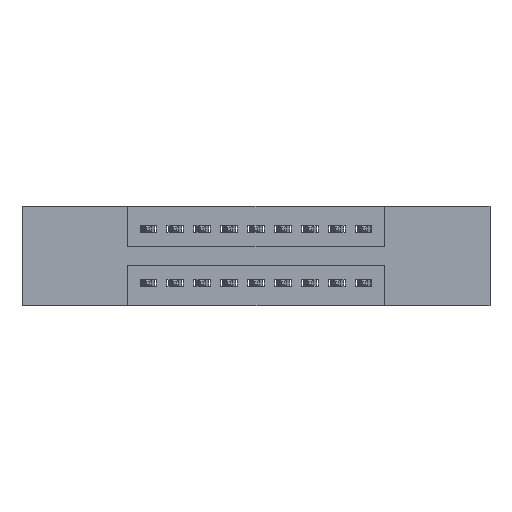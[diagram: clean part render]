
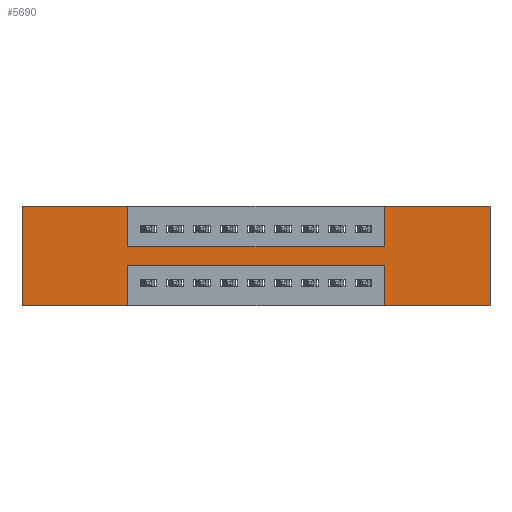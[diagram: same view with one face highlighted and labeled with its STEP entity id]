
A CAD part, front view. The second image highlights one B-rep face of the part: STEP entity #5690.
In plain terms, the highlighted planar face has unit normal (0, -1, 0).
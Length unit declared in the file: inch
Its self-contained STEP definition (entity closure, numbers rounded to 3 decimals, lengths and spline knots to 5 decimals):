
#27 = EDGE_CURVE ( 'NONE', #7362, #11286, #8275, .T. ) ;
#112 = VERTEX_POINT ( 'NONE', #4151 ) ;
#224 = LINE ( 'NONE', #10759, #5105 ) ;
#239 = VECTOR ( 'NONE', #3613, 39.37008 ) ;
#330 = LINE ( 'NONE', #7866, #8213 ) ;
#507 = CARTESIAN_POINT ( 'NONE',  ( 1.735, 0., -0.37 ) ) ;
#945 = VERTEX_POINT ( 'NONE', #2384 ) ;
#1227 = VERTEX_POINT ( 'NONE', #5487 ) ;
#1236 = ORIENTED_EDGE ( 'NONE', *, *, #6368, .F. ) ;
#1239 = LINE ( 'NONE', #10356, #7208 ) ;
#1295 = ORIENTED_EDGE ( 'NONE', *, *, #3933, .F. ) ;
#1447 = DIRECTION ( 'NONE',  ( -1., 0., 0. ) ) ;
#1628 = ORIENTED_EDGE ( 'NONE', *, *, #2714, .F. ) ;
#1631 = ORIENTED_EDGE ( 'NONE', *, *, #1986, .F. ) ;
#1646 = DIRECTION ( 'NONE',  ( 0., -1., 0. ) ) ;
#1829 = ORIENTED_EDGE ( 'NONE', *, *, #4329, .F. ) ;
#1986 = EDGE_CURVE ( 'NONE', #8914, #5612, #5753, .T. ) ;
#2113 = EDGE_CURVE ( 'NONE', #112, #8914, #330, .T. ) ;
#2194 = ORIENTED_EDGE ( 'NONE', *, *, #6553, .F. ) ;
#2314 = CARTESIAN_POINT ( 'NONE',  ( 0., 0., 0. ) ) ;
#2384 = CARTESIAN_POINT ( 'NONE',  ( 0.3925, 0., 0. ) ) ;
#2404 = CARTESIAN_POINT ( 'NONE',  ( 0., 0., 0. ) ) ;
#2482 = LINE ( 'NONE', #10685, #239 ) ;
#2489 = FACE_OUTER_BOUND ( 'NONE', #9531, .T. ) ;
#2555 = CARTESIAN_POINT ( 'NONE',  ( 1.3425, 0., -0.37 ) ) ;
#2714 = EDGE_CURVE ( 'NONE', #10929, #112, #3242, .T. ) ;
#2785 = VECTOR ( 'NONE', #1447, 39.37008 ) ;
#2789 = VERTEX_POINT ( 'NONE', #3865 ) ;
#2868 = ORIENTED_EDGE ( 'NONE', *, *, #27, .F. ) ;
#3043 = VECTOR ( 'NONE', #5498, 39.37008 ) ;
#3101 = CARTESIAN_POINT ( 'NONE',  ( 0.3925, 0., -0.22 ) ) ;
#3113 = CARTESIAN_POINT ( 'NONE',  ( 0., 0., -0.37 ) ) ;
#3242 = LINE ( 'NONE', #5253, #9728 ) ;
#3300 = DIRECTION ( 'NONE',  ( 0., 0., -1. ) ) ;
#3613 = DIRECTION ( 'NONE',  ( 0., 0., 1. ) ) ;
#3855 = ORIENTED_EDGE ( 'NONE', *, *, #9742, .F. ) ;
#3865 = CARTESIAN_POINT ( 'NONE',  ( 0.3925, 0., -0.15 ) ) ;
#3933 = EDGE_CURVE ( 'NONE', #945, #2789, #1239, .T. ) ;
#4038 = CARTESIAN_POINT ( 'NONE',  ( 0., 0., 0. ) ) ;
#4043 = LINE ( 'NONE', #9904, #5548 ) ;
#4151 = CARTESIAN_POINT ( 'NONE',  ( 0.3925, 0., -0.37 ) ) ;
#4329 = EDGE_CURVE ( 'NONE', #4394, #5399, #9144, .T. ) ;
#4394 = VERTEX_POINT ( 'NONE', #2555 ) ;
#4529 = EDGE_CURVE ( 'NONE', #5612, #945, #5687, .T. ) ;
#4893 = EDGE_CURVE ( 'NONE', #5399, #10929, #5140, .T. ) ;
#5105 = VECTOR ( 'NONE', #9064, 39.37008 ) ;
#5140 = LINE ( 'NONE', #10385, #2785 ) ;
#5190 = DIRECTION ( 'NONE',  ( 0., 0., 1. ) ) ;
#5253 = CARTESIAN_POINT ( 'NONE',  ( 0.3925, 0., -0.37 ) ) ;
#5386 = CARTESIAN_POINT ( 'NONE',  ( 1.735, 0., 0. ) ) ;
#5399 = VERTEX_POINT ( 'NONE', #8584 ) ;
#5487 = CARTESIAN_POINT ( 'NONE',  ( 1.3425, 0., -0.15 ) ) ;
#5498 = DIRECTION ( 'NONE',  ( 1., 0., 0. ) ) ;
#5548 = VECTOR ( 'NONE', #8063, 39.37008 ) ;
#5612 = VERTEX_POINT ( 'NONE', #4038 ) ;
#5619 = DIRECTION ( 'NONE',  ( 0., 0., 1. ) ) ;
#5687 = LINE ( 'NONE', #2314, #8302 ) ;
#5690 = ADVANCED_FACE ( 'NONE', ( #2489 ), #11340, .T. ) ;
#5753 = LINE ( 'NONE', #2404, #6993 ) ;
#6368 = EDGE_CURVE ( 'NONE', #1227, #7362, #2482, .T. ) ;
#6553 = EDGE_CURVE ( 'NONE', #9097, #4394, #224, .T. ) ;
#6993 = VECTOR ( 'NONE', #5190, 39.37008 ) ;
#7103 = DIRECTION ( 'NONE',  ( 1., 0., 0. ) ) ;
#7208 = VECTOR ( 'NONE', #3300, 39.37008 ) ;
#7300 = CARTESIAN_POINT ( 'NONE',  ( 1.3425, 0., -0.37 ) ) ;
#7362 = VERTEX_POINT ( 'NONE', #10953 ) ;
#7866 = CARTESIAN_POINT ( 'NONE',  ( 0., 0., -0.37 ) ) ;
#8063 = DIRECTION ( 'NONE',  ( 0., 0., -1. ) ) ;
#8213 = VECTOR ( 'NONE', #9744, 39.37008 ) ;
#8275 = LINE ( 'NONE', #8725, #3043 ) ;
#8302 = VECTOR ( 'NONE', #8568, 39.37008 ) ;
#8515 = ORIENTED_EDGE ( 'NONE', *, *, #4893, .F. ) ;
#8568 = DIRECTION ( 'NONE',  ( 1., 0., 0. ) ) ;
#8584 = CARTESIAN_POINT ( 'NONE',  ( 1.3425, 0., -0.22 ) ) ;
#8654 = EDGE_CURVE ( 'NONE', #11286, #9097, #4043, .T. ) ;
#8697 = CARTESIAN_POINT ( 'NONE',  ( 0., 0., -0.37 ) ) ;
#8725 = CARTESIAN_POINT ( 'NONE',  ( 0., 0., 0. ) ) ;
#8833 = VECTOR ( 'NONE', #7103, 39.37008 ) ;
#8914 = VERTEX_POINT ( 'NONE', #3113 ) ;
#9005 = VECTOR ( 'NONE', #5619, 39.37008 ) ;
#9064 = DIRECTION ( 'NONE',  ( -1., 0., 0. ) ) ;
#9097 = VERTEX_POINT ( 'NONE', #507 ) ;
#9144 = LINE ( 'NONE', #7300, #9005 ) ;
#9531 = EDGE_LOOP ( 'NONE', ( #1628, #8515, #1829, #2194, #11287, #2868, #1236, #3855, #1295, #11160, #1631, #11211 ) ) ;
#9689 = LINE ( 'NONE', #9712, #8833 ) ;
#9712 = CARTESIAN_POINT ( 'NONE',  ( 0.3925, 0., -0.15 ) ) ;
#9728 = VECTOR ( 'NONE', #10626, 39.37008 ) ;
#9742 = EDGE_CURVE ( 'NONE', #2789, #1227, #9689, .T. ) ;
#9744 = DIRECTION ( 'NONE',  ( -1., 0., 0. ) ) ;
#9904 = CARTESIAN_POINT ( 'NONE',  ( 1.735, 0., 0. ) ) ;
#10249 = AXIS2_PLACEMENT_3D ( 'NONE', #8697, #1646, #11417 ) ;
#10356 = CARTESIAN_POINT ( 'NONE',  ( 0.3925, 0., 0. ) ) ;
#10385 = CARTESIAN_POINT ( 'NONE',  ( 0.3925, 0., -0.22 ) ) ;
#10626 = DIRECTION ( 'NONE',  ( 0., 0., -1. ) ) ;
#10685 = CARTESIAN_POINT ( 'NONE',  ( 1.3425, 0., 0. ) ) ;
#10759 = CARTESIAN_POINT ( 'NONE',  ( 0., 0., -0.37 ) ) ;
#10929 = VERTEX_POINT ( 'NONE', #3101 ) ;
#10953 = CARTESIAN_POINT ( 'NONE',  ( 1.3425, 0., 0. ) ) ;
#11160 = ORIENTED_EDGE ( 'NONE', *, *, #4529, .F. ) ;
#11211 = ORIENTED_EDGE ( 'NONE', *, *, #2113, .F. ) ;
#11286 = VERTEX_POINT ( 'NONE', #5386 ) ;
#11287 = ORIENTED_EDGE ( 'NONE', *, *, #8654, .F. ) ;
#11340 = PLANE ( 'NONE',  #10249 ) ;
#11417 = DIRECTION ( 'NONE',  ( 0., 0., -1. ) ) ;
